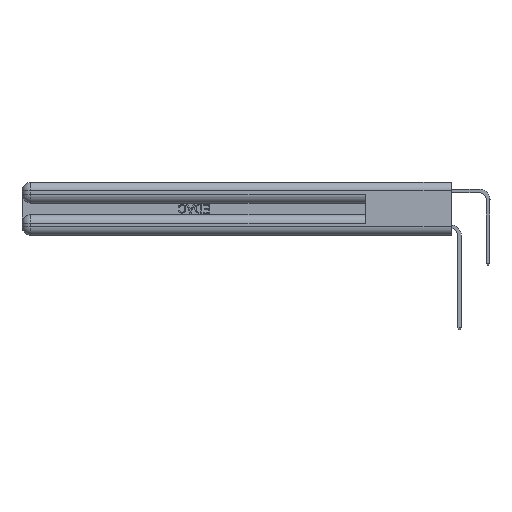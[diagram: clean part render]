
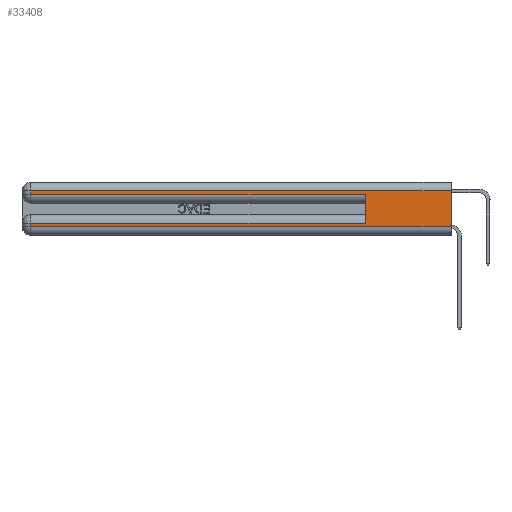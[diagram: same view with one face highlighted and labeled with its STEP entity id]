
A CAD part, left-side view. The second image highlights one B-rep face of the part: STEP entity #33408.
In plain terms, the highlighted planar face has unit normal (-1, 0, 0).
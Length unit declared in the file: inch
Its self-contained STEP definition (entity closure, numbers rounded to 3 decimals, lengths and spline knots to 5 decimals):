
#39 = DIRECTION ( 'NONE',  ( 0., 1., 0. ) ) ;
#1953 = EDGE_CURVE ( 'NONE', #8381, #37703, #2059, .T. ) ;
#2059 = LINE ( 'NONE', #22429, #30524 ) ;
#2735 = CARTESIAN_POINT ( 'NONE',  ( 0., 2.94, 0.285 ) ) ;
#3809 = CARTESIAN_POINT ( 'NONE',  ( 0., 0.6, 0.145 ) ) ;
#5096 = VECTOR ( 'NONE', #19466, 39.37008 ) ;
#5251 = DIRECTION ( 'NONE',  ( 0., -1., 0. ) ) ;
#6594 = ORIENTED_EDGE ( 'NONE', *, *, #14372, .T. ) ;
#6697 = CARTESIAN_POINT ( 'NONE',  ( 0., 0., 0.31 ) ) ;
#7171 = VECTOR ( 'NONE', #17184, 39.37008 ) ;
#7318 = CARTESIAN_POINT ( 'NONE',  ( 0., 0.6, 0.285 ) ) ;
#8164 = CARTESIAN_POINT ( 'NONE',  ( 0., 2.94, 0.06 ) ) ;
#8190 = VERTEX_POINT ( 'NONE', #8164 ) ;
#8238 = ORIENTED_EDGE ( 'NONE', *, *, #15189, .T. ) ;
#8381 = VERTEX_POINT ( 'NONE', #36148 ) ;
#8644 = ORIENTED_EDGE ( 'NONE', *, *, #1953, .T. ) ;
#8754 = DIRECTION ( 'NONE',  ( 0., -1., 0. ) ) ;
#9412 = LINE ( 'NONE', #3809, #29589 ) ;
#9810 = DIRECTION ( 'NONE',  ( 0., 1., 0. ) ) ;
#9834 = CARTESIAN_POINT ( 'NONE',  ( 0., 2.94, 0.085 ) ) ;
#10604 = EDGE_LOOP ( 'NONE', ( #32598, #21035, #8644, #35052, #15593, #14280, #8238, #6594 ) ) ;
#10676 = VERTEX_POINT ( 'NONE', #6697 ) ;
#11748 = AXIS2_PLACEMENT_3D ( 'NONE', #28421, #13810, #25724 ) ;
#12756 = VECTOR ( 'NONE', #39, 39.37008 ) ;
#12848 = DIRECTION ( 'NONE',  ( 0., 0., -1. ) ) ;
#13368 = VECTOR ( 'NONE', #9810, 39.37008 ) ;
#13810 = DIRECTION ( 'NONE',  ( 1., 0., 0. ) ) ;
#14255 = CARTESIAN_POINT ( 'NONE',  ( 0., 2.94, 0.37 ) ) ;
#14280 = ORIENTED_EDGE ( 'NONE', *, *, #28437, .T. ) ;
#14372 = EDGE_CURVE ( 'NONE', #8190, #34213, #24294, .T. ) ;
#14723 = CARTESIAN_POINT ( 'NONE',  ( 0., 0., 0.31 ) ) ;
#14879 = FACE_OUTER_BOUND ( 'NONE', #10604, .T. ) ;
#15189 = EDGE_CURVE ( 'NONE', #25233, #8190, #20963, .T. ) ;
#15593 = ORIENTED_EDGE ( 'NONE', *, *, #19269, .F. ) ;
#16626 = PLANE ( 'NONE',  #11748 ) ;
#17184 = DIRECTION ( 'NONE',  ( 0., 0., -1. ) ) ;
#17382 = LINE ( 'NONE', #14723, #12756 ) ;
#17602 = EDGE_CURVE ( 'NONE', #37703, #35598, #33879, .T. ) ;
#19269 = EDGE_CURVE ( 'NONE', #21973, #35598, #9412, .T. ) ;
#19466 = DIRECTION ( 'NONE',  ( 0., 0., -1. ) ) ;
#20963 = LINE ( 'NONE', #14255, #7171 ) ;
#21035 = ORIENTED_EDGE ( 'NONE', *, *, #31178, .T. ) ;
#21973 = VERTEX_POINT ( 'NONE', #37027 ) ;
#22429 = CARTESIAN_POINT ( 'NONE',  ( 0., 2.94, 0.37 ) ) ;
#22662 = CARTESIAN_POINT ( 'NONE',  ( 0., 0., 0.37 ) ) ;
#24294 = LINE ( 'NONE', #37988, #28866 ) ;
#25233 = VERTEX_POINT ( 'NONE', #9834 ) ;
#25724 = DIRECTION ( 'NONE',  ( 0., 0., -1. ) ) ;
#26202 = LINE ( 'NONE', #33120, #13368 ) ;
#26816 = CARTESIAN_POINT ( 'NONE',  ( 0., 0., 0.06 ) ) ;
#27016 = CARTESIAN_POINT ( 'NONE',  ( 0., 0., 0.285 ) ) ;
#28421 = CARTESIAN_POINT ( 'NONE',  ( 0., 0., 0.37 ) ) ;
#28437 = EDGE_CURVE ( 'NONE', #21973, #25233, #26202, .T. ) ;
#28866 = VECTOR ( 'NONE', #8754, 39.37008 ) ;
#29088 = DIRECTION ( 'NONE',  ( 0., 0., 1. ) ) ;
#29589 = VECTOR ( 'NONE', #29088, 39.37008 ) ;
#30524 = VECTOR ( 'NONE', #12848, 39.37008 ) ;
#31178 = EDGE_CURVE ( 'NONE', #10676, #8381, #17382, .T. ) ;
#32598 = ORIENTED_EDGE ( 'NONE', *, *, #37495, .F. ) ;
#32929 = VECTOR ( 'NONE', #5251, 39.37008 ) ;
#33120 = CARTESIAN_POINT ( 'NONE',  ( 0., 0., 0.085 ) ) ;
#33408 = ADVANCED_FACE ( 'NONE', ( #14879 ), #16626, .F. ) ;
#33879 = LINE ( 'NONE', #27016, #32929 ) ;
#34213 = VERTEX_POINT ( 'NONE', #26816 ) ;
#35052 = ORIENTED_EDGE ( 'NONE', *, *, #17602, .T. ) ;
#35390 = LINE ( 'NONE', #22662, #5096 ) ;
#35598 = VERTEX_POINT ( 'NONE', #7318 ) ;
#36148 = CARTESIAN_POINT ( 'NONE',  ( 0., 2.94, 0.31 ) ) ;
#37027 = CARTESIAN_POINT ( 'NONE',  ( 0., 0.6, 0.085 ) ) ;
#37495 = EDGE_CURVE ( 'NONE', #10676, #34213, #35390, .T. ) ;
#37703 = VERTEX_POINT ( 'NONE', #2735 ) ;
#37988 = CARTESIAN_POINT ( 'NONE',  ( 0., 0., 0.06 ) ) ;
